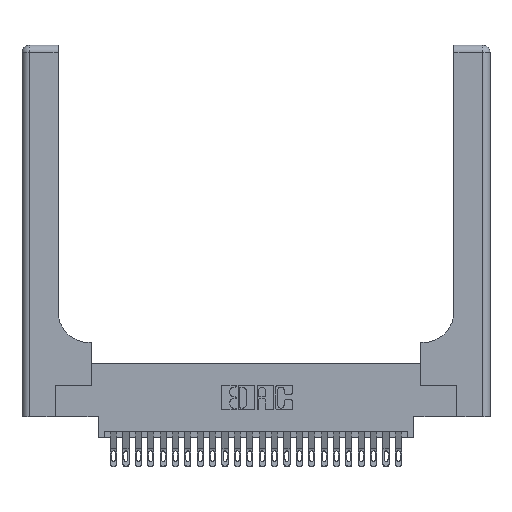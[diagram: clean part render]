
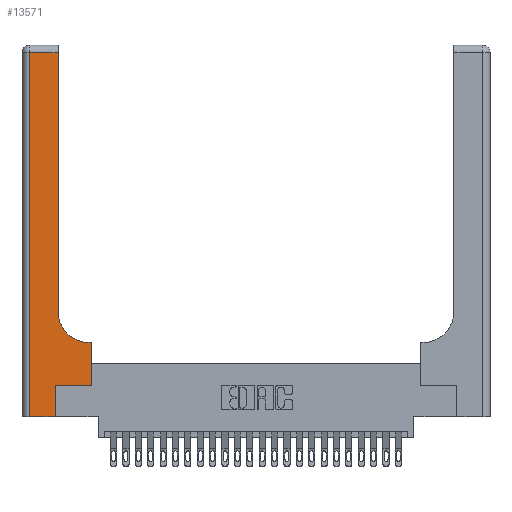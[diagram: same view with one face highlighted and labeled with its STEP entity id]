
A CAD part, top view. The second image highlights one B-rep face of the part: STEP entity #13571.
In plain terms, the highlighted planar face has unit normal (0, 0, 1).
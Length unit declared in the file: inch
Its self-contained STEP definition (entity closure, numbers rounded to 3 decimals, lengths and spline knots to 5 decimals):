
#418 = ORIENTED_EDGE ( 'NONE', *, *, #10270, .T. ) ;
#1130 = CARTESIAN_POINT ( 'NONE',  ( 0.2915, 3., 0.37 ) ) ;
#1298 = CIRCLE ( 'NONE', #24777, 0.25 ) ;
#1785 = LINE ( 'NONE', #25066, #17441 ) ;
#1841 = EDGE_CURVE ( 'NONE', #22903, #13937, #5898, .T. ) ;
#2128 = CARTESIAN_POINT ( 'NONE',  ( 0.2915, 2.94, 0.37 ) ) ;
#2247 = CARTESIAN_POINT ( 'NONE',  ( 0.2915, 0.85, 0.37 ) ) ;
#2302 = DIRECTION ( 'NONE',  ( 1., 0., 0. ) ) ;
#2341 = CARTESIAN_POINT ( 'NONE',  ( 0., 3., 0.37 ) ) ;
#2358 = VERTEX_POINT ( 'NONE', #11964 ) ;
#2474 = DIRECTION ( 'NONE',  ( 0., 1., 0. ) ) ;
#2481 = DIRECTION ( 'NONE',  ( 0., 0., -1. ) ) ;
#2757 = AXIS2_PLACEMENT_3D ( 'NONE', #2341, #20956, #4368 ) ;
#3018 = EDGE_LOOP ( 'NONE', ( #6656, #5302, #9615, #8754, #18654, #418, #10713, #26473, #21979 ) ) ;
#3407 = DIRECTION ( 'NONE',  ( 1., 0., 0. ) ) ;
#3479 = CARTESIAN_POINT ( 'NONE',  ( 0.06, 3., 0.37 ) ) ;
#4291 = VERTEX_POINT ( 'NONE', #7308 ) ;
#4368 = DIRECTION ( 'NONE',  ( -1., 0., 0. ) ) ;
#5302 = ORIENTED_EDGE ( 'NONE', *, *, #11648, .T. ) ;
#5742 = VERTEX_POINT ( 'NONE', #26363 ) ;
#5857 = DIRECTION ( 'NONE',  ( 0., 1., 0. ) ) ;
#5894 = EDGE_CURVE ( 'NONE', #2358, #4291, #21630, .T. ) ;
#5898 = LINE ( 'NONE', #1130, #15714 ) ;
#6449 = CARTESIAN_POINT ( 'NONE',  ( 0.5415, 0.85, 0.37 ) ) ;
#6656 = ORIENTED_EDGE ( 'NONE', *, *, #1841, .T. ) ;
#7308 = CARTESIAN_POINT ( 'NONE',  ( 0.5585, 0.6, 0.37 ) ) ;
#7312 = VERTEX_POINT ( 'NONE', #26183 ) ;
#8754 = ORIENTED_EDGE ( 'NONE', *, *, #16658, .T. ) ;
#9615 = ORIENTED_EDGE ( 'NONE', *, *, #14129, .T. ) ;
#9735 = CARTESIAN_POINT ( 'NONE',  ( 0., 0., 0.37 ) ) ;
#9740 = VECTOR ( 'NONE', #23468, 39.37008 ) ;
#9854 = LINE ( 'NONE', #15336, #19255 ) ;
#10270 = EDGE_CURVE ( 'NONE', #10496, #2358, #15265, .T. ) ;
#10496 = VERTEX_POINT ( 'NONE', #12565 ) ;
#10713 = ORIENTED_EDGE ( 'NONE', *, *, #5894, .T. ) ;
#11648 = EDGE_CURVE ( 'NONE', #13937, #21225, #1785, .T. ) ;
#11901 = EDGE_CURVE ( 'NONE', #5742, #10496, #20817, .T. ) ;
#11964 = CARTESIAN_POINT ( 'NONE',  ( 0.5585, 0.25, 0.37 ) ) ;
#12339 = CARTESIAN_POINT ( 'NONE',  ( 0.269, 0., 0.37 ) ) ;
#12565 = CARTESIAN_POINT ( 'NONE',  ( 0.269, 0.25, 0.37 ) ) ;
#12672 = DIRECTION ( 'NONE',  ( -1., 0., 0. ) ) ;
#13094 = CARTESIAN_POINT ( 'NONE',  ( 0.5585, 0.25, 0.37 ) ) ;
#13571 = ADVANCED_FACE ( 'NONE', ( #23313 ), #16706, .F. ) ;
#13937 = VERTEX_POINT ( 'NONE', #2128 ) ;
#14129 = EDGE_CURVE ( 'NONE', #21225, #15384, #19425, .T. ) ;
#15108 = VECTOR ( 'NONE', #3407, 39.37008 ) ;
#15265 = LINE ( 'NONE', #15535, #9740 ) ;
#15336 = CARTESIAN_POINT ( 'NONE',  ( 0.2915, 0.6, 0.37 ) ) ;
#15384 = VERTEX_POINT ( 'NONE', #22899 ) ;
#15535 = CARTESIAN_POINT ( 'NONE',  ( 0.269, 0.25, 0.37 ) ) ;
#15714 = VECTOR ( 'NONE', #15977, 39.37008 ) ;
#15977 = DIRECTION ( 'NONE',  ( 0., 1., 0. ) ) ;
#16658 = EDGE_CURVE ( 'NONE', #15384, #5742, #26412, .T. ) ;
#16706 = PLANE ( 'NONE',  #2757 ) ;
#17441 = VECTOR ( 'NONE', #12672, 39.37008 ) ;
#17895 = EDGE_CURVE ( 'NONE', #7312, #22903, #1298, .T. ) ;
#18654 = ORIENTED_EDGE ( 'NONE', *, *, #11901, .T. ) ;
#19255 = VECTOR ( 'NONE', #19571, 39.37008 ) ;
#19425 = LINE ( 'NONE', #3479, #20747 ) ;
#19571 = DIRECTION ( 'NONE',  ( -1., 0., 0. ) ) ;
#19861 = VECTOR ( 'NONE', #5857, 39.37008 ) ;
#20466 = DIRECTION ( 'NONE',  ( 0., -1., 0. ) ) ;
#20747 = VECTOR ( 'NONE', #20466, 39.37008 ) ;
#20817 = LINE ( 'NONE', #12339, #19861 ) ;
#20956 = DIRECTION ( 'NONE',  ( 0., 0., -1. ) ) ;
#21225 = VERTEX_POINT ( 'NONE', #23736 ) ;
#21630 = LINE ( 'NONE', #13094, #22586 ) ;
#21979 = ORIENTED_EDGE ( 'NONE', *, *, #17895, .T. ) ;
#22586 = VECTOR ( 'NONE', #2474, 39.37008 ) ;
#22899 = CARTESIAN_POINT ( 'NONE',  ( 0.06, 0., 0.37 ) ) ;
#22903 = VERTEX_POINT ( 'NONE', #2247 ) ;
#23313 = FACE_OUTER_BOUND ( 'NONE', #3018, .T. ) ;
#23468 = DIRECTION ( 'NONE',  ( 1., 0., 0. ) ) ;
#23736 = CARTESIAN_POINT ( 'NONE',  ( 0.06, 2.94, 0.37 ) ) ;
#24777 = AXIS2_PLACEMENT_3D ( 'NONE', #6449, #2481, #2302 ) ;
#25066 = CARTESIAN_POINT ( 'NONE',  ( 0., 2.94, 0.37 ) ) ;
#25881 = EDGE_CURVE ( 'NONE', #4291, #7312, #9854, .T. ) ;
#26183 = CARTESIAN_POINT ( 'NONE',  ( 0.5415, 0.6, 0.37 ) ) ;
#26363 = CARTESIAN_POINT ( 'NONE',  ( 0.269, 0., 0.37 ) ) ;
#26412 = LINE ( 'NONE', #9735, #15108 ) ;
#26473 = ORIENTED_EDGE ( 'NONE', *, *, #25881, .T. ) ;
